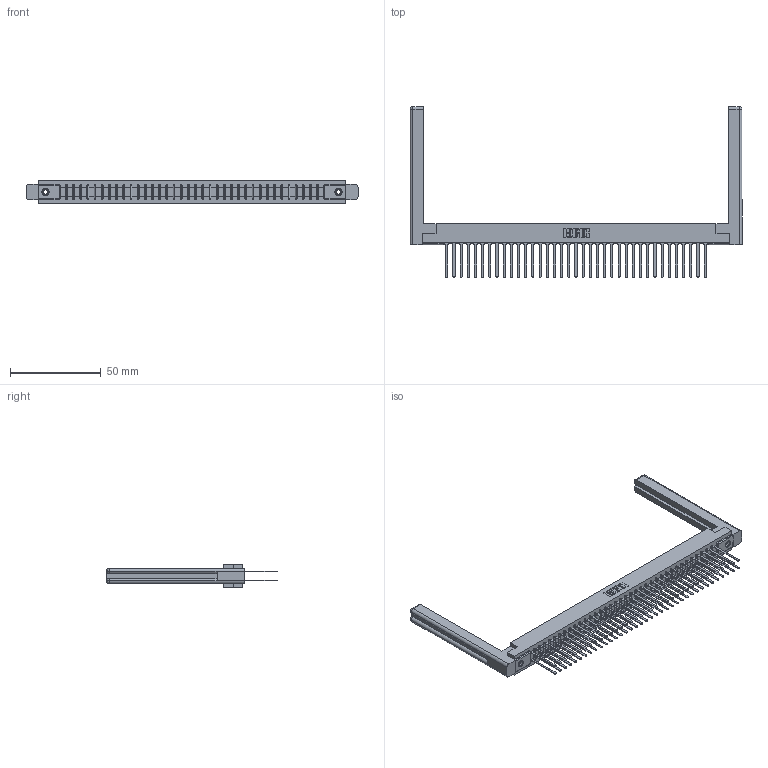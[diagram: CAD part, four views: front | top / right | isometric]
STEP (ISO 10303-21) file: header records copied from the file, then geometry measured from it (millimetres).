
FILE_DESCRIPTION (( 'STEP AP203' ), '1' );
FILE_NAME ('357-074-440-258.STEP', '2020-10-04T17:41:44', ( '' ), ( '' ), 'SwSTEP 2.0', 'SolidWorks 2020', '' );
FILE_SCHEMA (( 'CONFIG_CONTROL_DESIGN' ));
Length unit declared in the file: inch
Products named in the file (5): 307-290-001_540; 307 Part_.156 Dia Mounting Holes; 345-250-001_345-250-001-102; 307-220-058; 357-074-440-258
Assembly tree (79 placements, depth 2):
  357-074-440-258
    307 Part_.156 Dia Mounting Holes
    307-290-001_540  x74
    307-220-058  x2
    345-250-001_345-250-001-102  x2
Bounding box: 183.24 x 94.31 x 12.7 mm (x, y, z)
Volume: 26992.1 mm3; surface area: 31564 mm2
Topology: 79 solids, 79 shells, 3702 faces, 10297 edges, 6650 vertices
Faces by surface type: plane 2448, cylinder 1154, sphere 76, torus 12, cone 12
Entity records: 36121 total; most frequent: CARTESIAN_POINT 5928, ORIENTED_EDGE 5816, DIRECTION 5766, EDGE_CURVE 2908, VECTOR 2226, LINE 2226, VERTEX_POINT 1878, AXIS2_PLACEMENT_3D 1770
